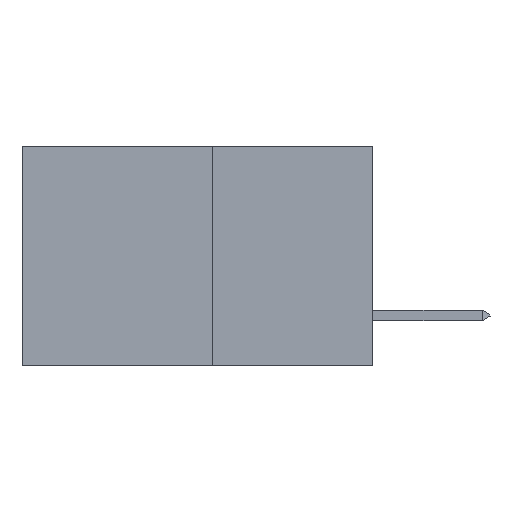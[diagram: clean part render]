
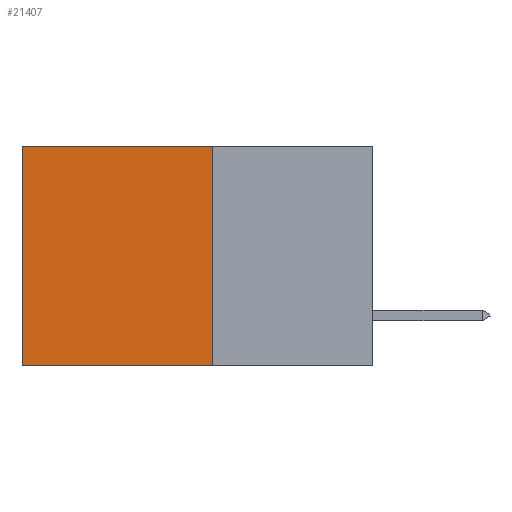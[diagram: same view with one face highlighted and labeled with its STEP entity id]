
A CAD part, left-side view. The second image highlights one B-rep face of the part: STEP entity #21407.
In plain terms, the highlighted planar face has unit normal (-1, 0, 0).
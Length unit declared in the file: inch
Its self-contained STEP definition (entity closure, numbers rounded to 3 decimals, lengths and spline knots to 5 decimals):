
#816 = CARTESIAN_POINT ( 'NONE',  ( 0.277, 0.59, 0. ) ) ;
#1098 = CARTESIAN_POINT ( 'NONE',  ( 0.277, 0.27, 0. ) ) ;
#2109 = ORIENTED_EDGE ( 'NONE', *, *, #18815, .T. ) ;
#2910 = ORIENTED_EDGE ( 'NONE', *, *, #14877, .T. ) ;
#3015 = DIRECTION ( 'NONE',  ( 0., 1., 0. ) ) ;
#4268 = VERTEX_POINT ( 'NONE', #7933 ) ;
#4367 = LINE ( 'NONE', #1098, #8887 ) ;
#4603 = DIRECTION ( 'NONE',  ( 0., 1., 0. ) ) ;
#5168 = DIRECTION ( 'NONE',  ( 0., 0., -1. ) ) ;
#5352 = VECTOR ( 'NONE', #5168, 39.37008 ) ;
#6398 = AXIS2_PLACEMENT_3D ( 'NONE', #8865, #20707, #10588 ) ;
#7933 = CARTESIAN_POINT ( 'NONE',  ( 0.277, 0.27, -0.37 ) ) ;
#8565 = VERTEX_POINT ( 'NONE', #816 ) ;
#8865 = CARTESIAN_POINT ( 'NONE',  ( 0.277, 0.27, -0.37 ) ) ;
#8887 = VECTOR ( 'NONE', #4603, 39.37008 ) ;
#10041 = VECTOR ( 'NONE', #3015, 39.37008 ) ;
#10120 = EDGE_CURVE ( 'NONE', #4268, #11506, #14531, .T. ) ;
#10588 = DIRECTION ( 'NONE',  ( 0., 0., -1. ) ) ;
#11506 = VERTEX_POINT ( 'NONE', #17963 ) ;
#11530 = CARTESIAN_POINT ( 'NONE',  ( 0.277, 0.27, 0. ) ) ;
#12257 = VERTEX_POINT ( 'NONE', #11530 ) ;
#13515 = EDGE_LOOP ( 'NONE', ( #2910, #17078, #18689, #2109 ) ) ;
#14531 = LINE ( 'NONE', #14903, #10041 ) ;
#14877 = EDGE_CURVE ( 'NONE', #8565, #11506, #19394, .T. ) ;
#14903 = CARTESIAN_POINT ( 'NONE',  ( 0.277, 0.27, -0.37 ) ) ;
#15348 = CARTESIAN_POINT ( 'NONE',  ( 0.277, 0.59, -0.37 ) ) ;
#16579 = VECTOR ( 'NONE', #17159, 39.37008 ) ;
#17078 = ORIENTED_EDGE ( 'NONE', *, *, #10120, .F. ) ;
#17082 = CARTESIAN_POINT ( 'NONE',  ( 0.277, 0.27, -0.37 ) ) ;
#17159 = DIRECTION ( 'NONE',  ( 0., 0., -1. ) ) ;
#17963 = CARTESIAN_POINT ( 'NONE',  ( 0.277, 0.59, -0.37 ) ) ;
#18689 = ORIENTED_EDGE ( 'NONE', *, *, #19039, .F. ) ;
#18815 = EDGE_CURVE ( 'NONE', #12257, #8565, #4367, .T. ) ;
#19039 = EDGE_CURVE ( 'NONE', #12257, #4268, #21022, .T. ) ;
#19049 = PLANE ( 'NONE',  #6398 ) ;
#19394 = LINE ( 'NONE', #15348, #5352 ) ;
#20604 = FACE_OUTER_BOUND ( 'NONE', #13515, .T. ) ;
#20707 = DIRECTION ( 'NONE',  ( 1., 0., 0. ) ) ;
#21022 = LINE ( 'NONE', #17082, #16579 ) ;
#21407 = ADVANCED_FACE ( 'NONE', ( #20604 ), #19049, .F. ) ;
